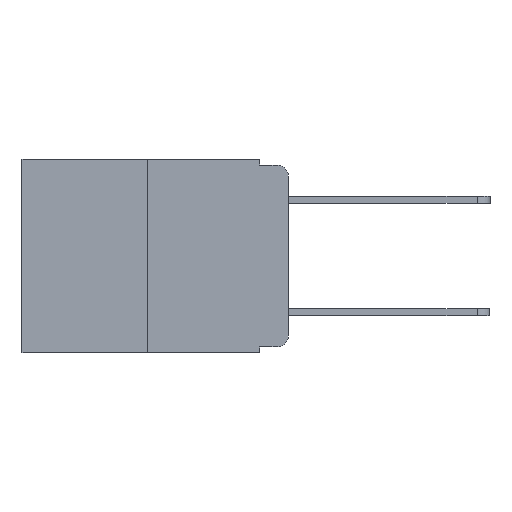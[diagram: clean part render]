
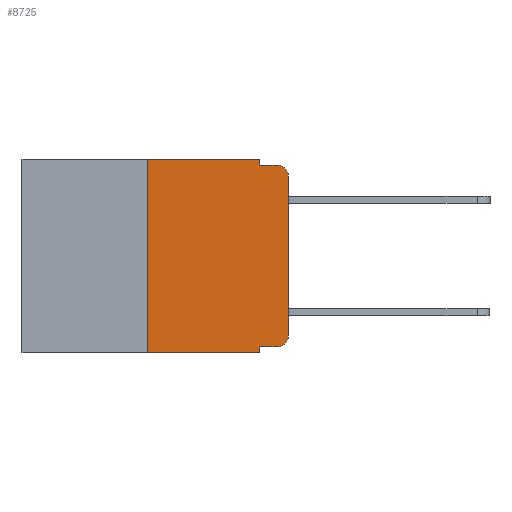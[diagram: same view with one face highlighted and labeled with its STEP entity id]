
A CAD part, left-side view. The second image highlights one B-rep face of the part: STEP entity #8725.
In plain terms, the highlighted planar face has unit normal (-1, 0, 0).
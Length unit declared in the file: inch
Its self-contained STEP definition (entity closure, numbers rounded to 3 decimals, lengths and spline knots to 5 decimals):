
#238 = CARTESIAN_POINT ( 'NONE',  ( 0., 0.473, 0. ) ) ;
#608 = LINE ( 'NONE', #19099, #5317 ) ;
#1218 = VECTOR ( 'NONE', #11537, 39.37008 ) ;
#1232 = VERTEX_POINT ( 'NONE', #5105 ) ;
#1713 = DIRECTION ( 'NONE',  ( 0., -1., 0. ) ) ;
#1737 = DIRECTION ( 'NONE',  ( 0., 0., 1. ) ) ;
#1770 = CARTESIAN_POINT ( 'NONE',  ( 0., 0., -0.03 ) ) ;
#2668 = EDGE_LOOP ( 'NONE', ( #17477, #21220, #7091, #5577, #11292, #13107, #21239, #17589, #18841, #4670 ) ) ;
#2885 = CARTESIAN_POINT ( 'NONE',  ( 0., 0.473, -0.343 ) ) ;
#3154 = AXIS2_PLACEMENT_3D ( 'NONE', #14809, #3252, #16732 ) ;
#3252 = DIRECTION ( 'NONE',  ( -1., 0., 0. ) ) ;
#3262 = EDGE_CURVE ( 'NONE', #5961, #10813, #6683, .T. ) ;
#3269 = LINE ( 'NONE', #17016, #23132 ) ;
#3778 = CARTESIAN_POINT ( 'NONE',  ( 0., 0., 0. ) ) ;
#3915 = EDGE_CURVE ( 'NONE', #14070, #15204, #6346, .T. ) ;
#4052 = EDGE_CURVE ( 'NONE', #1232, #21603, #3269, .T. ) ;
#4075 = LINE ( 'NONE', #15303, #7437 ) ;
#4418 = CARTESIAN_POINT ( 'NONE',  ( 0., 0.051, -0.343 ) ) ;
#4577 = EDGE_CURVE ( 'NONE', #11111, #23918, #11706, .T. ) ;
#4670 = ORIENTED_EDGE ( 'NONE', *, *, #3262, .T. ) ;
#4943 = VERTEX_POINT ( 'NONE', #6307 ) ;
#5097 = DIRECTION ( 'NONE',  ( -1., 0., 0. ) ) ;
#5105 = CARTESIAN_POINT ( 'NONE',  ( 0., 0.051, 0. ) ) ;
#5317 = VECTOR ( 'NONE', #1737, 39.37008 ) ;
#5392 = EDGE_CURVE ( 'NONE', #21603, #15204, #15795, .T. ) ;
#5457 = CARTESIAN_POINT ( 'NONE',  ( 0., 0., -0.313 ) ) ;
#5512 = DIRECTION ( 'NONE',  ( 0., 0., -1. ) ) ;
#5577 = ORIENTED_EDGE ( 'NONE', *, *, #4052, .F. ) ;
#5596 = DIRECTION ( 'NONE',  ( 0., -1., 0. ) ) ;
#5840 = LINE ( 'NONE', #12730, #15462 ) ;
#5961 = VERTEX_POINT ( 'NONE', #8650 ) ;
#6307 = CARTESIAN_POINT ( 'NONE',  ( 0., 0.25, 0. ) ) ;
#6346 = CIRCLE ( 'NONE', #19471, 0.02 ) ;
#6433 = CARTESIAN_POINT ( 'NONE',  ( 0., 0.051, -0.333 ) ) ;
#6683 = CIRCLE ( 'NONE', #3154, 0.02 ) ;
#7091 = ORIENTED_EDGE ( 'NONE', *, *, #5392, .F. ) ;
#7185 = CARTESIAN_POINT ( 'NONE',  ( 0., 0.051, -0.01 ) ) ;
#7437 = VECTOR ( 'NONE', #1713, 39.37008 ) ;
#8596 = DIRECTION ( 'NONE',  ( 1., 0., 0. ) ) ;
#8650 = CARTESIAN_POINT ( 'NONE',  ( 0., 0.02, -0.333 ) ) ;
#8725 = ADVANCED_FACE ( 'NONE', ( #21640 ), #16214, .F. ) ;
#10096 = VECTOR ( 'NONE', #5596, 39.37008 ) ;
#10813 = VERTEX_POINT ( 'NONE', #5457 ) ;
#11111 = VERTEX_POINT ( 'NONE', #21748 ) ;
#11292 = ORIENTED_EDGE ( 'NONE', *, *, #24536, .F. ) ;
#11537 = DIRECTION ( 'NONE',  ( 0., 0., 1. ) ) ;
#11706 = LINE ( 'NONE', #2885, #16815 ) ;
#12059 = DIRECTION ( 'NONE',  ( 0., -1., 0. ) ) ;
#12525 = DIRECTION ( 'NONE',  ( 0., -1., 0. ) ) ;
#12730 = CARTESIAN_POINT ( 'NONE',  ( 0., 0.051, 0. ) ) ;
#12776 = VECTOR ( 'NONE', #12059, 39.37008 ) ;
#13107 = ORIENTED_EDGE ( 'NONE', *, *, #16977, .F. ) ;
#14055 = CARTESIAN_POINT ( 'NONE',  ( 0., 0.02, -0.01 ) ) ;
#14070 = VERTEX_POINT ( 'NONE', #1770 ) ;
#14671 = DIRECTION ( 'NONE',  ( 0., 0., -1. ) ) ;
#14809 = CARTESIAN_POINT ( 'NONE',  ( 0., 0.02, -0.313 ) ) ;
#15204 = VERTEX_POINT ( 'NONE', #14055 ) ;
#15303 = CARTESIAN_POINT ( 'NONE',  ( 0., 0.051, -0.333 ) ) ;
#15462 = VECTOR ( 'NONE', #14671, 39.37008 ) ;
#15795 = LINE ( 'NONE', #22820, #10096 ) ;
#16214 = PLANE ( 'NONE',  #24959 ) ;
#16617 = CARTESIAN_POINT ( 'NONE',  ( 0., 0.02, -0.03 ) ) ;
#16732 = DIRECTION ( 'NONE',  ( 0., 0., -1. ) ) ;
#16815 = VECTOR ( 'NONE', #12525, 39.37008 ) ;
#16977 = EDGE_CURVE ( 'NONE', #11111, #4943, #608, .T. ) ;
#17016 = CARTESIAN_POINT ( 'NONE',  ( 0., 0.051, 0. ) ) ;
#17477 = ORIENTED_EDGE ( 'NONE', *, *, #19093, .T. ) ;
#17589 = ORIENTED_EDGE ( 'NONE', *, *, #24670, .F. ) ;
#17840 = LINE ( 'NONE', #238, #12776 ) ;
#17881 = VERTEX_POINT ( 'NONE', #6433 ) ;
#18263 = EDGE_CURVE ( 'NONE', #17881, #5961, #4075, .T. ) ;
#18549 = DIRECTION ( 'NONE',  ( 0., 0., -1. ) ) ;
#18841 = ORIENTED_EDGE ( 'NONE', *, *, #18263, .T. ) ;
#19093 = EDGE_CURVE ( 'NONE', #10813, #14070, #20633, .T. ) ;
#19099 = CARTESIAN_POINT ( 'NONE',  ( 0., 0.25, 0. ) ) ;
#19471 = AXIS2_PLACEMENT_3D ( 'NONE', #16617, #5097, #18549 ) ;
#20081 = CARTESIAN_POINT ( 'NONE',  ( 0., 0.473, 0. ) ) ;
#20633 = LINE ( 'NONE', #3778, #1218 ) ;
#21220 = ORIENTED_EDGE ( 'NONE', *, *, #3915, .T. ) ;
#21239 = ORIENTED_EDGE ( 'NONE', *, *, #4577, .T. ) ;
#21603 = VERTEX_POINT ( 'NONE', #7185 ) ;
#21640 = FACE_OUTER_BOUND ( 'NONE', #2668, .T. ) ;
#21748 = CARTESIAN_POINT ( 'NONE',  ( 0., 0.25, -0.343 ) ) ;
#22015 = DIRECTION ( 'NONE',  ( 0., 0., -1. ) ) ;
#22820 = CARTESIAN_POINT ( 'NONE',  ( 0., 0.051, -0.01 ) ) ;
#23132 = VECTOR ( 'NONE', #5512, 39.37008 ) ;
#23918 = VERTEX_POINT ( 'NONE', #4418 ) ;
#24536 = EDGE_CURVE ( 'NONE', #4943, #1232, #17840, .T. ) ;
#24670 = EDGE_CURVE ( 'NONE', #17881, #23918, #5840, .T. ) ;
#24959 = AXIS2_PLACEMENT_3D ( 'NONE', #20081, #8596, #22015 ) ;
